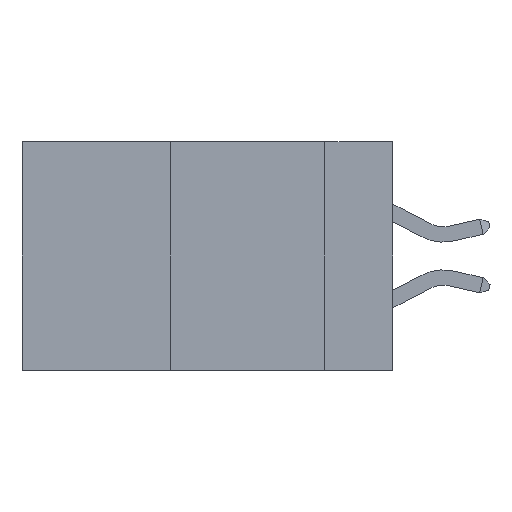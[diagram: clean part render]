
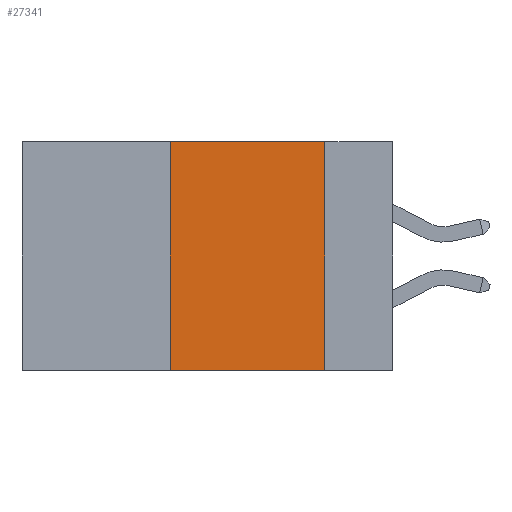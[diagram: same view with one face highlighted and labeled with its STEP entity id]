
A CAD part, left-side view. The second image highlights one B-rep face of the part: STEP entity #27341.
In plain terms, the highlighted planar face has unit normal (-1, 0, 0).
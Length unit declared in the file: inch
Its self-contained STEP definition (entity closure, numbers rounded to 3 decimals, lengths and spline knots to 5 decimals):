
#217 = LINE ( 'NONE', #38761, #6456 ) ;
#977 = CARTESIAN_POINT ( 'NONE',  ( 0., 0.36, -0.37 ) ) ;
#1538 = VECTOR ( 'NONE', #27757, 39.37008 ) ;
#6456 = VECTOR ( 'NONE', #20326, 39.37008 ) ;
#6850 = LINE ( 'NONE', #33026, #1538 ) ;
#7946 = DIRECTION ( 'NONE',  ( 1., 0., 0. ) ) ;
#8006 = FACE_OUTER_BOUND ( 'NONE', #29714, .T. ) ;
#9379 = DIRECTION ( 'NONE',  ( 0., -1., 0. ) ) ;
#9445 = VECTOR ( 'NONE', #22849, 39.37008 ) ;
#10889 = LINE ( 'NONE', #37673, #9445 ) ;
#12229 = ORIENTED_EDGE ( 'NONE', *, *, #35360, .T. ) ;
#15648 = CARTESIAN_POINT ( 'NONE',  ( 0., 0.11, -0.37 ) ) ;
#15834 = VERTEX_POINT ( 'NONE', #15648 ) ;
#19035 = AXIS2_PLACEMENT_3D ( 'NONE', #23404, #7946, #29464 ) ;
#20326 = DIRECTION ( 'NONE',  ( 0., 0., -1. ) ) ;
#22369 = CARTESIAN_POINT ( 'NONE',  ( 0., 0.36, 0. ) ) ;
#22571 = VERTEX_POINT ( 'NONE', #22369 ) ;
#22849 = DIRECTION ( 'NONE',  ( 0., 0., 1. ) ) ;
#23404 = CARTESIAN_POINT ( 'NONE',  ( 0., 0.6, 0. ) ) ;
#24032 = EDGE_CURVE ( 'NONE', #22571, #28556, #6850, .T. ) ;
#26565 = ORIENTED_EDGE ( 'NONE', *, *, #27315, .F. ) ;
#27281 = ORIENTED_EDGE ( 'NONE', *, *, #30578, .F. ) ;
#27315 = EDGE_CURVE ( 'NONE', #32877, #22571, #10889, .T. ) ;
#27341 = ADVANCED_FACE ( 'NONE', ( #8006 ), #32565, .F. ) ;
#27757 = DIRECTION ( 'NONE',  ( 0., -1., 0. ) ) ;
#27957 = ORIENTED_EDGE ( 'NONE', *, *, #24032, .F. ) ;
#28556 = VERTEX_POINT ( 'NONE', #37454 ) ;
#29464 = DIRECTION ( 'NONE',  ( 0., 0., -1. ) ) ;
#29714 = EDGE_LOOP ( 'NONE', ( #27281, #27957, #26565, #12229 ) ) ;
#30578 = EDGE_CURVE ( 'NONE', #28556, #15834, #217, .T. ) ;
#32565 = PLANE ( 'NONE',  #19035 ) ;
#32877 = VERTEX_POINT ( 'NONE', #977 ) ;
#33026 = CARTESIAN_POINT ( 'NONE',  ( 0., 0.6, 0. ) ) ;
#34018 = CARTESIAN_POINT ( 'NONE',  ( 0., 0.6, -0.37 ) ) ;
#35360 = EDGE_CURVE ( 'NONE', #32877, #15834, #38658, .T. ) ;
#37454 = CARTESIAN_POINT ( 'NONE',  ( 0., 0.11, 0. ) ) ;
#37673 = CARTESIAN_POINT ( 'NONE',  ( 0., 0.36, 0. ) ) ;
#38658 = LINE ( 'NONE', #34018, #39161 ) ;
#38761 = CARTESIAN_POINT ( 'NONE',  ( 0., 0.11, 0. ) ) ;
#39161 = VECTOR ( 'NONE', #9379, 39.37008 ) ;
